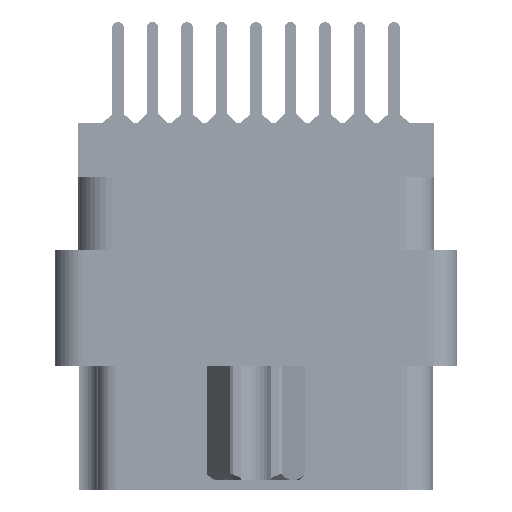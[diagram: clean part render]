
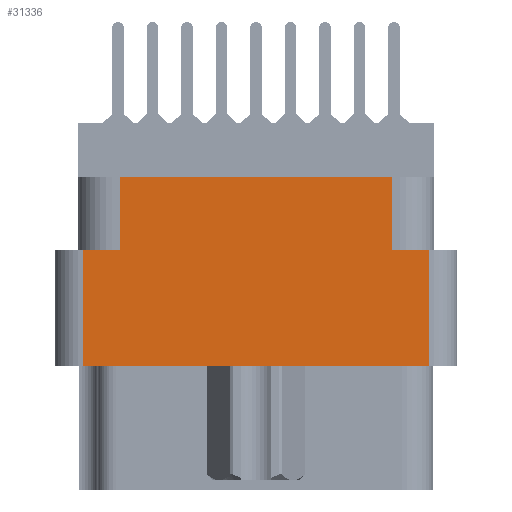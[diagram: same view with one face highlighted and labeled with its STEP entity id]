
A CAD part, left-side view. The second image highlights one B-rep face of the part: STEP entity #31336.
In plain terms, the highlighted planar face has unit normal (-1, 0, 0).
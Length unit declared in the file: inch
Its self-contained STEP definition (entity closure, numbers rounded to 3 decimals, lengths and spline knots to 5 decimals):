
#911 = VECTOR ( 'NONE', #21689, 39.37008 ) ;
#992 = CARTESIAN_POINT ( 'NONE',  ( -1.296, 0.376, -0.798 ) ) ;
#3308 = VERTEX_POINT ( 'NONE', #36085 ) ;
#4055 = VERTEX_POINT ( 'NONE', #47386 ) ;
#4927 = VECTOR ( 'NONE', #50864, 39.37008 ) ;
#5029 = DIRECTION ( 'NONE',  ( 0., -1., 0. ) ) ;
#5753 = ORIENTED_EDGE ( 'NONE', *, *, #58630, .F. ) ;
#7171 = VERTEX_POINT ( 'NONE', #58324 ) ;
#7177 = CARTESIAN_POINT ( 'NONE',  ( -1.296, 0., -0.277 ) ) ;
#7236 = EDGE_CURVE ( 'NONE', #7171, #56658, #25442, .T. ) ;
#7352 = VECTOR ( 'NONE', #29490, 39.37008 ) ;
#7605 = EDGE_CURVE ( 'NONE', #17428, #45429, #53674, .T. ) ;
#7704 = ORIENTED_EDGE ( 'NONE', *, *, #34785, .F. ) ;
#8679 = CARTESIAN_POINT ( 'NONE',  ( -1.296, -0.438, -0.798 ) ) ;
#8876 = CARTESIAN_POINT ( 'NONE',  ( -1.296, 0.376, -0.529 ) ) ;
#9291 = DIRECTION ( 'NONE',  ( 0., -1., 0. ) ) ;
#9702 = ORIENTED_EDGE ( 'NONE', *, *, #7605, .F. ) ;
#10728 = VECTOR ( 'NONE', #9291, 39.37008 ) ;
#11115 = CARTESIAN_POINT ( 'NONE',  ( -1.296, -0.376, -0.277 ) ) ;
#11202 = EDGE_CURVE ( 'NONE', #17428, #15424, #45420, .T. ) ;
#11943 = LINE ( 'NONE', #37740, #43070 ) ;
#12021 = CARTESIAN_POINT ( 'NONE',  ( -1.296, -0.296, -0.277 ) ) ;
#12945 = EDGE_CURVE ( 'NONE', #17667, #45429, #47055, .T. ) ;
#14952 = CARTESIAN_POINT ( 'NONE',  ( -1.296, -0.296, -0.117 ) ) ;
#15424 = VERTEX_POINT ( 'NONE', #11115 ) ;
#16891 = EDGE_CURVE ( 'NONE', #4055, #56658, #11943, .T. ) ;
#17428 = VERTEX_POINT ( 'NONE', #32435 ) ;
#17556 = PLANE ( 'NONE',  #41725 ) ;
#17607 = VECTOR ( 'NONE', #39350, 39.37008 ) ;
#17667 = VERTEX_POINT ( 'NONE', #20848 ) ;
#20848 = CARTESIAN_POINT ( 'NONE',  ( -1.296, 0.376, -0.277 ) ) ;
#21689 = DIRECTION ( 'NONE',  ( 0., 0., 1. ) ) ;
#25442 = LINE ( 'NONE', #12021, #911 ) ;
#25809 = ORIENTED_EDGE ( 'NONE', *, *, #7236, .T. ) ;
#29490 = DIRECTION ( 'NONE',  ( 0., 1., 0. ) ) ;
#31336 = ADVANCED_FACE ( 'NONE', ( #44070 ), #17556, .T. ) ;
#32435 = CARTESIAN_POINT ( 'NONE',  ( -1.296, -0.376, -0.529 ) ) ;
#33297 = DIRECTION ( 'NONE',  ( 0., 0., -1. ) ) ;
#33501 = CARTESIAN_POINT ( 'NONE',  ( -1.296, 0., -0.529 ) ) ;
#34785 = EDGE_CURVE ( 'NONE', #7171, #15424, #45844, .T. ) ;
#35975 = DIRECTION ( 'NONE',  ( -1., 0., 0. ) ) ;
#36085 = CARTESIAN_POINT ( 'NONE',  ( -1.296, 0.296, -0.277 ) ) ;
#37740 = CARTESIAN_POINT ( 'NONE',  ( -1.296, 0.438, -0.117 ) ) ;
#38535 = EDGE_CURVE ( 'NONE', #3308, #4055, #48477, .T. ) ;
#39350 = DIRECTION ( 'NONE',  ( 0., -1., 0. ) ) ;
#41480 = ORIENTED_EDGE ( 'NONE', *, *, #38535, .F. ) ;
#41725 = AXIS2_PLACEMENT_3D ( 'NONE', #8679, #35975, #59447 ) ;
#41787 = EDGE_LOOP ( 'NONE', ( #5753, #53107, #9702, #42352, #7704, #25809, #48292, #41480 ) ) ;
#42277 = CARTESIAN_POINT ( 'NONE',  ( -1.296, 0.296, -0.277 ) ) ;
#42352 = ORIENTED_EDGE ( 'NONE', *, *, #11202, .T. ) ;
#43070 = VECTOR ( 'NONE', #5029, 39.37008 ) ;
#44070 = FACE_OUTER_BOUND ( 'NONE', #41787, .T. ) ;
#45420 = LINE ( 'NONE', #46218, #4927 ) ;
#45429 = VERTEX_POINT ( 'NONE', #8876 ) ;
#45844 = LINE ( 'NONE', #7177, #17607 ) ;
#46100 = CARTESIAN_POINT ( 'NONE',  ( -1.296, 0., -0.277 ) ) ;
#46218 = CARTESIAN_POINT ( 'NONE',  ( -1.296, -0.376, -0.798 ) ) ;
#46367 = VECTOR ( 'NONE', #33297, 39.37008 ) ;
#47055 = LINE ( 'NONE', #992, #46367 ) ;
#47386 = CARTESIAN_POINT ( 'NONE',  ( -1.296, 0.296, -0.117 ) ) ;
#48292 = ORIENTED_EDGE ( 'NONE', *, *, #16891, .F. ) ;
#48477 = LINE ( 'NONE', #42277, #52082 ) ;
#49080 = LINE ( 'NONE', #46100, #10728 ) ;
#50864 = DIRECTION ( 'NONE',  ( 0., 0., 1. ) ) ;
#52082 = VECTOR ( 'NONE', #56228, 39.37008 ) ;
#53107 = ORIENTED_EDGE ( 'NONE', *, *, #12945, .T. ) ;
#53674 = LINE ( 'NONE', #33501, #7352 ) ;
#56228 = DIRECTION ( 'NONE',  ( 0., 0., 1. ) ) ;
#56658 = VERTEX_POINT ( 'NONE', #14952 ) ;
#58324 = CARTESIAN_POINT ( 'NONE',  ( -1.296, -0.296, -0.277 ) ) ;
#58630 = EDGE_CURVE ( 'NONE', #17667, #3308, #49080, .T. ) ;
#59447 = DIRECTION ( 'NONE',  ( 0., 0., 1. ) ) ;
